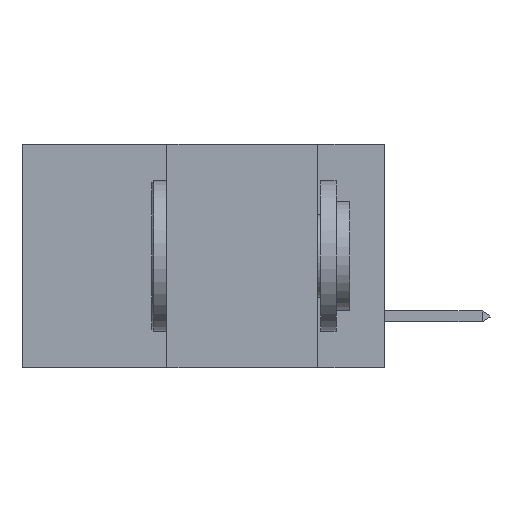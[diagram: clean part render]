
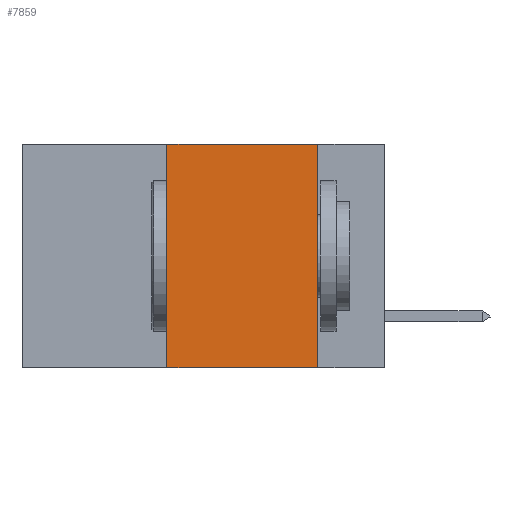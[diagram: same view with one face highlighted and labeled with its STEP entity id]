
A CAD part, left-side view. The second image highlights one B-rep face of the part: STEP entity #7859.
In plain terms, the highlighted planar face has unit normal (-1, 0, 0).
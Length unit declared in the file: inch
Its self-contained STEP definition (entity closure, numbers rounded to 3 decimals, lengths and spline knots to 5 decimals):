
#1290 = EDGE_CURVE ( 'NONE', #8323, #8674, #31649, .T. ) ;
#3402 = DIRECTION ( 'NONE',  ( 0., -1., 0. ) ) ;
#3789 = CARTESIAN_POINT ( 'NONE',  ( 0., 0.6, 0. ) ) ;
#4742 = CARTESIAN_POINT ( 'NONE',  ( 0., 0.36, 0. ) ) ;
#4865 = CARTESIAN_POINT ( 'NONE',  ( 0., 0.11, 0. ) ) ;
#6620 = VERTEX_POINT ( 'NONE', #32487 ) ;
#7561 = LINE ( 'NONE', #4865, #22808 ) ;
#7597 = CARTESIAN_POINT ( 'NONE',  ( 0., 0.36, 0. ) ) ;
#7859 = ADVANCED_FACE ( 'NONE', ( #22229 ), #33402, .F. ) ;
#8323 = VERTEX_POINT ( 'NONE', #8984 ) ;
#8674 = VERTEX_POINT ( 'NONE', #4742 ) ;
#8924 = EDGE_CURVE ( 'NONE', #8323, #6620, #15400, .T. ) ;
#8984 = CARTESIAN_POINT ( 'NONE',  ( 0., 0.36, -0.37 ) ) ;
#9438 = ORIENTED_EDGE ( 'NONE', *, *, #22867, .F. ) ;
#9602 = EDGE_LOOP ( 'NONE', ( #9438, #34373, #33536, #12665 ) ) ;
#10265 = VECTOR ( 'NONE', #14794, 39.37008 ) ;
#11994 = DIRECTION ( 'NONE',  ( 1., 0., 0. ) ) ;
#12493 = EDGE_CURVE ( 'NONE', #8674, #30831, #17970, .T. ) ;
#12665 = ORIENTED_EDGE ( 'NONE', *, *, #8924, .T. ) ;
#13388 = CARTESIAN_POINT ( 'NONE',  ( 0., 0.11, 0. ) ) ;
#14052 = CARTESIAN_POINT ( 'NONE',  ( 0., 0.6, -0.37 ) ) ;
#14377 = DIRECTION ( 'NONE',  ( 0., 0., -1. ) ) ;
#14534 = VECTOR ( 'NONE', #3402, 39.37008 ) ;
#14794 = DIRECTION ( 'NONE',  ( 0., -1., 0. ) ) ;
#15148 = VECTOR ( 'NONE', #29388, 39.37008 ) ;
#15400 = LINE ( 'NONE', #14052, #14534 ) ;
#17970 = LINE ( 'NONE', #3789, #10265 ) ;
#22229 = FACE_OUTER_BOUND ( 'NONE', #9602, .T. ) ;
#22808 = VECTOR ( 'NONE', #34616, 39.37008 ) ;
#22867 = EDGE_CURVE ( 'NONE', #30831, #6620, #7561, .T. ) ;
#27882 = CARTESIAN_POINT ( 'NONE',  ( 0., 0.6, 0. ) ) ;
#29388 = DIRECTION ( 'NONE',  ( 0., 0., 1. ) ) ;
#30664 = AXIS2_PLACEMENT_3D ( 'NONE', #27882, #11994, #14377 ) ;
#30831 = VERTEX_POINT ( 'NONE', #13388 ) ;
#31649 = LINE ( 'NONE', #7597, #15148 ) ;
#32487 = CARTESIAN_POINT ( 'NONE',  ( 0., 0.11, -0.37 ) ) ;
#33402 = PLANE ( 'NONE',  #30664 ) ;
#33536 = ORIENTED_EDGE ( 'NONE', *, *, #1290, .F. ) ;
#34373 = ORIENTED_EDGE ( 'NONE', *, *, #12493, .F. ) ;
#34616 = DIRECTION ( 'NONE',  ( 0., 0., -1. ) ) ;
